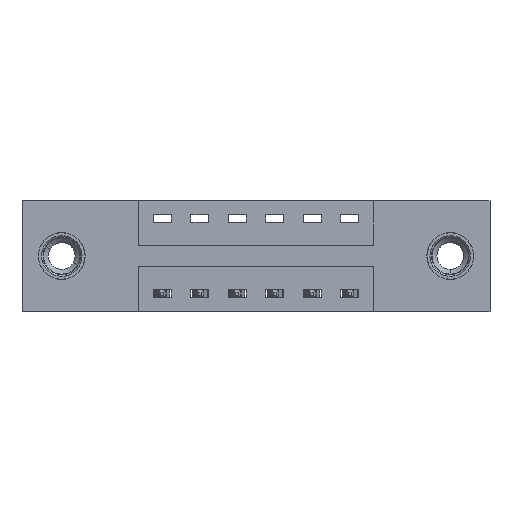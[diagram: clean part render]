
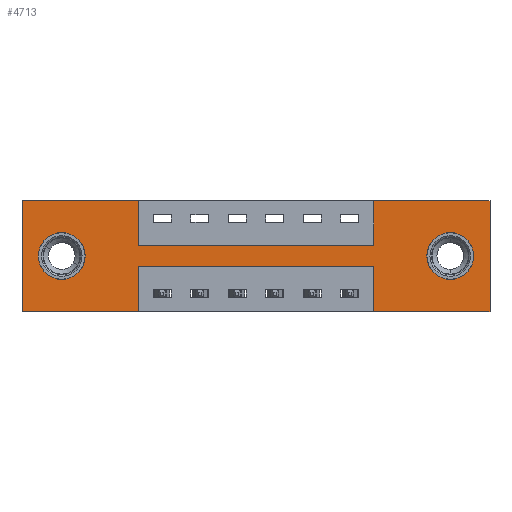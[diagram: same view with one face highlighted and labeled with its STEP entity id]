
A CAD part, front view. The second image highlights one B-rep face of the part: STEP entity #4713.
In plain terms, the highlighted planar face has unit normal (0, -1, 0).
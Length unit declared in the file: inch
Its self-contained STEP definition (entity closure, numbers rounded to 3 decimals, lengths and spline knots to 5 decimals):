
#32 = CARTESIAN_POINT ( 'NONE',  ( 0.3875, 0., 0. ) ) ;
#42 = AXIS2_PLACEMENT_3D ( 'NONE', #9432, #4917, #386 ) ;
#59 = ORIENTED_EDGE ( 'NONE', *, *, #3597, .F. ) ;
#116 = VECTOR ( 'NONE', #5698, 39.37008 ) ;
#156 = EDGE_CURVE ( 'NONE', #968, #3816, #9309, .T. ) ;
#160 = CARTESIAN_POINT ( 'NONE',  ( 1.56, 0., 0. ) ) ;
#201 = VERTEX_POINT ( 'NONE', #8671 ) ;
#296 = EDGE_CURVE ( 'NONE', #3219, #3259, #4345, .T. ) ;
#314 = ORIENTED_EDGE ( 'NONE', *, *, #2140, .F. ) ;
#335 = VERTEX_POINT ( 'NONE', #5949 ) ;
#386 = DIRECTION ( 'NONE',  ( 0., 0., -1. ) ) ;
#418 = CARTESIAN_POINT ( 'NONE',  ( 0., 0., -0.37 ) ) ;
#439 = DIRECTION ( 'NONE',  ( 1., 0., 0. ) ) ;
#769 = CIRCLE ( 'NONE', #42, 0.078 ) ;
#821 = ORIENTED_EDGE ( 'NONE', *, *, #1743, .F. ) ;
#859 = LINE ( 'NONE', #7392, #8661 ) ;
#968 = VERTEX_POINT ( 'NONE', #1547 ) ;
#995 = CARTESIAN_POINT ( 'NONE',  ( 1.56, 0., 0. ) ) ;
#1113 = ORIENTED_EDGE ( 'NONE', *, *, #7641, .F. ) ;
#1115 = DIRECTION ( 'NONE',  ( 0., 0., 1. ) ) ;
#1138 = EDGE_CURVE ( 'NONE', #4300, #4478, #2553, .T. ) ;
#1151 = EDGE_LOOP ( 'NONE', ( #5362, #3801 ) ) ;
#1225 = LINE ( 'NONE', #2957, #5013 ) ;
#1227 = CARTESIAN_POINT ( 'NONE',  ( 1.1725, 0., 0. ) ) ;
#1270 = VERTEX_POINT ( 'NONE', #7917 ) ;
#1547 = CARTESIAN_POINT ( 'NONE',  ( 0.1325, 0., -0.107 ) ) ;
#1733 = CARTESIAN_POINT ( 'NONE',  ( 0., 0., 0. ) ) ;
#1743 = EDGE_CURVE ( 'NONE', #8638, #335, #9390, .T. ) ;
#1836 = DIRECTION ( 'NONE',  ( -1., 0., 0. ) ) ;
#1879 = CARTESIAN_POINT ( 'NONE',  ( 1.1725, 0., -0.37 ) ) ;
#1961 = VERTEX_POINT ( 'NONE', #8130 ) ;
#1972 = ORIENTED_EDGE ( 'NONE', *, *, #3116, .F. ) ;
#1997 = CARTESIAN_POINT ( 'NONE',  ( 0.3875, 0., -0.22 ) ) ;
#2039 = VERTEX_POINT ( 'NONE', #5945 ) ;
#2049 = EDGE_CURVE ( 'NONE', #2039, #2528, #1225, .T. ) ;
#2053 = VECTOR ( 'NONE', #5329, 39.37008 ) ;
#2054 = CIRCLE ( 'NONE', #7279, 0.078 ) ;
#2137 = LINE ( 'NONE', #418, #116 ) ;
#2140 = EDGE_CURVE ( 'NONE', #6409, #1961, #7838, .T. ) ;
#2253 = DIRECTION ( 'NONE',  ( 0., 0., -1. ) ) ;
#2471 = EDGE_LOOP ( 'NONE', ( #5642, #7436, #5783, #821, #7580, #5784, #9241, #8260, #314, #1113, #59, #1972 ) ) ;
#2528 = VERTEX_POINT ( 'NONE', #1227 ) ;
#2553 = CIRCLE ( 'NONE', #8562, 0.078 ) ;
#2580 = AXIS2_PLACEMENT_3D ( 'NONE', #4394, #9693, #5167 ) ;
#2601 = FACE_OUTER_BOUND ( 'NONE', #2471, .T. ) ;
#2618 = VECTOR ( 'NONE', #1115, 39.37008 ) ;
#2712 = LINE ( 'NONE', #6869, #8483 ) ;
#2802 = CARTESIAN_POINT ( 'NONE',  ( 1.1725, 0., -0.22 ) ) ;
#2957 = CARTESIAN_POINT ( 'NONE',  ( 1.1725, 0., 0. ) ) ;
#3034 = LINE ( 'NONE', #7529, #6822 ) ;
#3060 = EDGE_CURVE ( 'NONE', #335, #3219, #8639, .T. ) ;
#3116 = EDGE_CURVE ( 'NONE', #4888, #1270, #2137, .T. ) ;
#3219 = VERTEX_POINT ( 'NONE', #2802 ) ;
#3259 = VERTEX_POINT ( 'NONE', #6593 ) ;
#3265 = DIRECTION ( 'NONE',  ( 0., 1., 0. ) ) ;
#3358 = CARTESIAN_POINT ( 'NONE',  ( 0., 0., -0.37 ) ) ;
#3360 = VECTOR ( 'NONE', #1836, 39.37008 ) ;
#3432 = CARTESIAN_POINT ( 'NONE',  ( 0.3875, 0., 0. ) ) ;
#3597 = EDGE_CURVE ( 'NONE', #1270, #201, #8384, .T. ) ;
#3801 = ORIENTED_EDGE ( 'NONE', *, *, #1138, .T. ) ;
#3816 = VERTEX_POINT ( 'NONE', #5419 ) ;
#3880 = CARTESIAN_POINT ( 'NONE',  ( 1.56, 0., -0.37 ) ) ;
#3918 = VERTEX_POINT ( 'NONE', #995 ) ;
#3919 = VECTOR ( 'NONE', #6256, 39.37008 ) ;
#3970 = LINE ( 'NONE', #9489, #4199 ) ;
#4079 = CARTESIAN_POINT ( 'NONE',  ( 1.4275, 0., -0.107 ) ) ;
#4117 = VECTOR ( 'NONE', #7624, 39.37008 ) ;
#4199 = VECTOR ( 'NONE', #439, 39.37008 ) ;
#4300 = VERTEX_POINT ( 'NONE', #8992 ) ;
#4345 = LINE ( 'NONE', #1997, #4117 ) ;
#4394 = CARTESIAN_POINT ( 'NONE',  ( 0., 0., -0.37 ) ) ;
#4416 = ORIENTED_EDGE ( 'NONE', *, *, #7860, .T. ) ;
#4472 = DIRECTION ( 'NONE',  ( 0., 1., 0. ) ) ;
#4478 = VERTEX_POINT ( 'NONE', #4079 ) ;
#4582 = VECTOR ( 'NONE', #7735, 39.37008 ) ;
#4713 = ADVANCED_FACE ( 'NONE', ( #4835, #6610, #2601 ), #6662, .T. ) ;
#4835 = FACE_BOUND ( 'NONE', #1151, .T. ) ;
#4888 = VERTEX_POINT ( 'NONE', #6119 ) ;
#4917 = DIRECTION ( 'NONE',  ( 0., 1., 0. ) ) ;
#5013 = VECTOR ( 'NONE', #9010, 39.37008 ) ;
#5117 = DIRECTION ( 'NONE',  ( 1., 0., 0. ) ) ;
#5167 = DIRECTION ( 'NONE',  ( 0., 0., -1. ) ) ;
#5329 = DIRECTION ( 'NONE',  ( 0., 0., -1. ) ) ;
#5362 = ORIENTED_EDGE ( 'NONE', *, *, #6956, .T. ) ;
#5419 = CARTESIAN_POINT ( 'NONE',  ( 0.1325, 0., -0.263 ) ) ;
#5575 = AXIS2_PLACEMENT_3D ( 'NONE', #7035, #7486, #8070 ) ;
#5611 = EDGE_CURVE ( 'NONE', #3918, #8638, #8846, .T. ) ;
#5642 = ORIENTED_EDGE ( 'NONE', *, *, #6043, .F. ) ;
#5698 = DIRECTION ( 'NONE',  ( -1., 0., 0. ) ) ;
#5783 = ORIENTED_EDGE ( 'NONE', *, *, #3060, .F. ) ;
#5784 = ORIENTED_EDGE ( 'NONE', *, *, #8407, .F. ) ;
#5945 = CARTESIAN_POINT ( 'NONE',  ( 1.1725, 0., -0.15 ) ) ;
#5949 = CARTESIAN_POINT ( 'NONE',  ( 1.1725, 0., -0.37 ) ) ;
#6043 = EDGE_CURVE ( 'NONE', #3259, #4888, #3034, .T. ) ;
#6119 = CARTESIAN_POINT ( 'NONE',  ( 0.3875, 0., -0.37 ) ) ;
#6256 = DIRECTION ( 'NONE',  ( 0., 0., 1. ) ) ;
#6409 = VERTEX_POINT ( 'NONE', #3432 ) ;
#6593 = CARTESIAN_POINT ( 'NONE',  ( 0.3875, 0., -0.22 ) ) ;
#6610 = FACE_BOUND ( 'NONE', #9232, .T. ) ;
#6662 = PLANE ( 'NONE',  #2580 ) ;
#6790 = ORIENTED_EDGE ( 'NONE', *, *, #156, .T. ) ;
#6822 = VECTOR ( 'NONE', #2253, 39.37008 ) ;
#6869 = CARTESIAN_POINT ( 'NONE',  ( 0.3875, 0., -0.15 ) ) ;
#6956 = EDGE_CURVE ( 'NONE', #4478, #4300, #769, .T. ) ;
#7035 = CARTESIAN_POINT ( 'NONE',  ( 0.1325, 0., -0.185 ) ) ;
#7279 = AXIS2_PLACEMENT_3D ( 'NONE', #9003, #4472, #9743 ) ;
#7392 = CARTESIAN_POINT ( 'NONE',  ( 0., 0., 0. ) ) ;
#7436 = ORIENTED_EDGE ( 'NONE', *, *, #296, .F. ) ;
#7486 = DIRECTION ( 'NONE',  ( 0., 1., 0. ) ) ;
#7529 = CARTESIAN_POINT ( 'NONE',  ( 0.3875, 0., -0.37 ) ) ;
#7580 = ORIENTED_EDGE ( 'NONE', *, *, #5611, .F. ) ;
#7613 = DIRECTION ( 'NONE',  ( 1., 0., 0. ) ) ;
#7624 = DIRECTION ( 'NONE',  ( -1., 0., 0. ) ) ;
#7641 = EDGE_CURVE ( 'NONE', #201, #6409, #3970, .T. ) ;
#7735 = DIRECTION ( 'NONE',  ( 0., 0., -1. ) ) ;
#7787 = CARTESIAN_POINT ( 'NONE',  ( 1.4275, 0., -0.185 ) ) ;
#7838 = LINE ( 'NONE', #32, #2053 ) ;
#7860 = EDGE_CURVE ( 'NONE', #3816, #968, #2054, .T. ) ;
#7917 = CARTESIAN_POINT ( 'NONE',  ( 0., 0., -0.37 ) ) ;
#8070 = DIRECTION ( 'NONE',  ( 0., 0., 1. ) ) ;
#8130 = CARTESIAN_POINT ( 'NONE',  ( 0.3875, 0., -0.15 ) ) ;
#8260 = ORIENTED_EDGE ( 'NONE', *, *, #9143, .F. ) ;
#8384 = LINE ( 'NONE', #1733, #3919 ) ;
#8407 = EDGE_CURVE ( 'NONE', #2528, #3918, #859, .T. ) ;
#8483 = VECTOR ( 'NONE', #7613, 39.37008 ) ;
#8546 = DIRECTION ( 'NONE',  ( 0., 0., -1. ) ) ;
#8562 = AXIS2_PLACEMENT_3D ( 'NONE', #7787, #3265, #8546 ) ;
#8638 = VERTEX_POINT ( 'NONE', #3880 ) ;
#8639 = LINE ( 'NONE', #1879, #2618 ) ;
#8661 = VECTOR ( 'NONE', #5117, 39.37008 ) ;
#8671 = CARTESIAN_POINT ( 'NONE',  ( 0., 0., 0. ) ) ;
#8846 = LINE ( 'NONE', #160, #4582 ) ;
#8992 = CARTESIAN_POINT ( 'NONE',  ( 1.4275, 0., -0.263 ) ) ;
#9003 = CARTESIAN_POINT ( 'NONE',  ( 0.1325, 0., -0.185 ) ) ;
#9010 = DIRECTION ( 'NONE',  ( 0., 0., 1. ) ) ;
#9143 = EDGE_CURVE ( 'NONE', #1961, #2039, #2712, .T. ) ;
#9232 = EDGE_LOOP ( 'NONE', ( #6790, #4416 ) ) ;
#9241 = ORIENTED_EDGE ( 'NONE', *, *, #2049, .F. ) ;
#9309 = CIRCLE ( 'NONE', #5575, 0.078 ) ;
#9390 = LINE ( 'NONE', #3358, #3360 ) ;
#9432 = CARTESIAN_POINT ( 'NONE',  ( 1.4275, 0., -0.185 ) ) ;
#9489 = CARTESIAN_POINT ( 'NONE',  ( 0., 0., 0. ) ) ;
#9693 = DIRECTION ( 'NONE',  ( 0., -1., 0. ) ) ;
#9743 = DIRECTION ( 'NONE',  ( 0., 0., 1. ) ) ;
